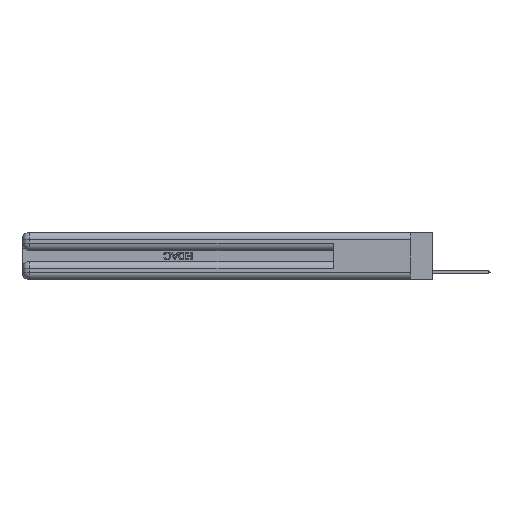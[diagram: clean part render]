
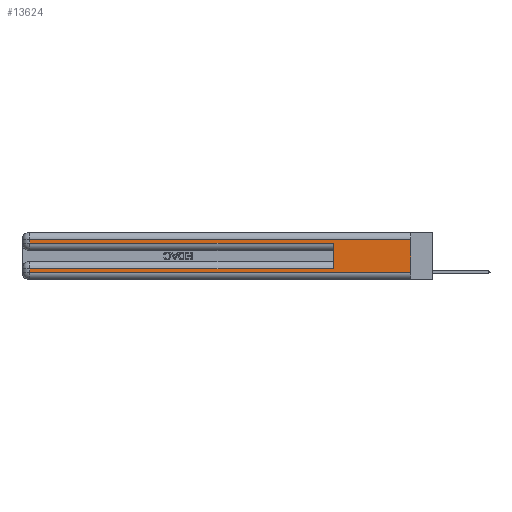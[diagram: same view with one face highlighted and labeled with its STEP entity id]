
A CAD part, left-side view. The second image highlights one B-rep face of the part: STEP entity #13624.
In plain terms, the highlighted planar face has unit normal (-1, 0, 0).
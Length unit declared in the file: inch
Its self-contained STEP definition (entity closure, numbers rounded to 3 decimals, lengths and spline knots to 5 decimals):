
#1159 = DIRECTION ( 'NONE',  ( 1., 0., 0. ) ) ;
#1387 = EDGE_CURVE ( 'NONE', #7971, #25365, #3560, .T. ) ;
#1438 = DIRECTION ( 'NONE',  ( 0., 0., -1. ) ) ;
#1611 = CARTESIAN_POINT ( 'NONE',  ( 0., 2.94, 0.37 ) ) ;
#2907 = DIRECTION ( 'NONE',  ( 0., 0., -1. ) ) ;
#2980 = LINE ( 'NONE', #29977, #3993 ) ;
#3402 = DIRECTION ( 'NONE',  ( 0., -1., 0. ) ) ;
#3560 = LINE ( 'NONE', #25332, #20906 ) ;
#3833 = VERTEX_POINT ( 'NONE', #22626 ) ;
#3993 = VECTOR ( 'NONE', #17881, 39.37008 ) ;
#5180 = CARTESIAN_POINT ( 'NONE',  ( 0., 0., 0.37 ) ) ;
#5302 = VECTOR ( 'NONE', #2907, 39.37008 ) ;
#5605 = ORIENTED_EDGE ( 'NONE', *, *, #6957, .T. ) ;
#6585 = DIRECTION ( 'NONE',  ( 0., 1., 0. ) ) ;
#6957 = EDGE_CURVE ( 'NONE', #27853, #15298, #10660, .T. ) ;
#7113 = CARTESIAN_POINT ( 'NONE',  ( 0., 0.6, 0.145 ) ) ;
#7971 = VERTEX_POINT ( 'NONE', #28167 ) ;
#8102 = VECTOR ( 'NONE', #28490, 39.37008 ) ;
#8666 = CARTESIAN_POINT ( 'NONE',  ( 0., 0.6, 0.085 ) ) ;
#8866 = ORIENTED_EDGE ( 'NONE', *, *, #13100, .T. ) ;
#8986 = CARTESIAN_POINT ( 'NONE',  ( 0., 0., 0.37 ) ) ;
#9442 = EDGE_CURVE ( 'NONE', #27853, #3833, #30385, .T. ) ;
#9568 = DIRECTION ( 'NONE',  ( 0., 0., 1. ) ) ;
#9670 = EDGE_CURVE ( 'NONE', #12974, #23420, #14510, .T. ) ;
#9767 = DIRECTION ( 'NONE',  ( 0., 0., -1. ) ) ;
#10368 = ORIENTED_EDGE ( 'NONE', *, *, #19626, .T. ) ;
#10532 = ORIENTED_EDGE ( 'NONE', *, *, #17558, .T. ) ;
#10660 = LINE ( 'NONE', #20659, #8102 ) ;
#10689 = CARTESIAN_POINT ( 'NONE',  ( 0., 2.94, 0.085 ) ) ;
#12111 = CARTESIAN_POINT ( 'NONE',  ( 0., 0.6, 0.285 ) ) ;
#12369 = LINE ( 'NONE', #7113, #12391 ) ;
#12391 = VECTOR ( 'NONE', #9568, 39.37008 ) ;
#12974 = VERTEX_POINT ( 'NONE', #10689 ) ;
#13100 = EDGE_CURVE ( 'NONE', #30931, #12974, #26408, .T. ) ;
#13624 = ADVANCED_FACE ( 'NONE', ( #18341 ), #28957, .F. ) ;
#14510 = LINE ( 'NONE', #1611, #22073 ) ;
#15298 = VERTEX_POINT ( 'NONE', #16345 ) ;
#15861 = ORIENTED_EDGE ( 'NONE', *, *, #9442, .F. ) ;
#15967 = ORIENTED_EDGE ( 'NONE', *, *, #18221, .F. ) ;
#16345 = CARTESIAN_POINT ( 'NONE',  ( 0., 2.94, 0.31 ) ) ;
#16576 = CARTESIAN_POINT ( 'NONE',  ( 0., 2.94, 0.06 ) ) ;
#17457 = EDGE_LOOP ( 'NONE', ( #15861, #5605, #10368, #26592, #15967, #8866, #30675, #10532 ) ) ;
#17558 = EDGE_CURVE ( 'NONE', #23420, #3833, #2980, .T. ) ;
#17881 = DIRECTION ( 'NONE',  ( 0., -1., 0. ) ) ;
#18221 = EDGE_CURVE ( 'NONE', #30931, #25365, #12369, .T. ) ;
#18341 = FACE_OUTER_BOUND ( 'NONE', #17457, .T. ) ;
#18897 = CARTESIAN_POINT ( 'NONE',  ( 0., 0., 0.31 ) ) ;
#19570 = VECTOR ( 'NONE', #6585, 39.37008 ) ;
#19626 = EDGE_CURVE ( 'NONE', #15298, #7971, #22232, .T. ) ;
#20659 = CARTESIAN_POINT ( 'NONE',  ( 0., 0., 0.31 ) ) ;
#20906 = VECTOR ( 'NONE', #3402, 39.37008 ) ;
#22073 = VECTOR ( 'NONE', #1438, 39.37008 ) ;
#22232 = LINE ( 'NONE', #32194, #32303 ) ;
#22626 = CARTESIAN_POINT ( 'NONE',  ( 0., 0., 0.06 ) ) ;
#22717 = AXIS2_PLACEMENT_3D ( 'NONE', #8986, #1159, #26021 ) ;
#23420 = VERTEX_POINT ( 'NONE', #16576 ) ;
#25332 = CARTESIAN_POINT ( 'NONE',  ( 0., 0., 0.285 ) ) ;
#25365 = VERTEX_POINT ( 'NONE', #12111 ) ;
#26021 = DIRECTION ( 'NONE',  ( 0., 0., -1. ) ) ;
#26408 = LINE ( 'NONE', #29330, #19570 ) ;
#26592 = ORIENTED_EDGE ( 'NONE', *, *, #1387, .T. ) ;
#27853 = VERTEX_POINT ( 'NONE', #18897 ) ;
#28167 = CARTESIAN_POINT ( 'NONE',  ( 0., 2.94, 0.285 ) ) ;
#28490 = DIRECTION ( 'NONE',  ( 0., 1., 0. ) ) ;
#28957 = PLANE ( 'NONE',  #22717 ) ;
#29330 = CARTESIAN_POINT ( 'NONE',  ( 0., 0., 0.085 ) ) ;
#29977 = CARTESIAN_POINT ( 'NONE',  ( 0., 0., 0.06 ) ) ;
#30385 = LINE ( 'NONE', #5180, #5302 ) ;
#30675 = ORIENTED_EDGE ( 'NONE', *, *, #9670, .T. ) ;
#30931 = VERTEX_POINT ( 'NONE', #8666 ) ;
#32194 = CARTESIAN_POINT ( 'NONE',  ( 0., 2.94, 0.37 ) ) ;
#32303 = VECTOR ( 'NONE', #9767, 39.37008 ) ;
